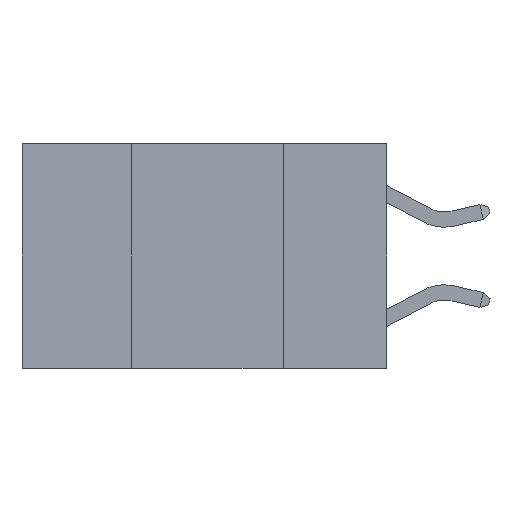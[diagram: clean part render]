
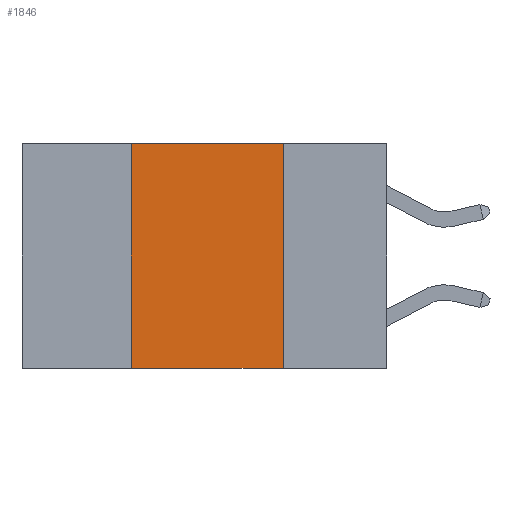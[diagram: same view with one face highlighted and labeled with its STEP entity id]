
A CAD part, left-side view. The second image highlights one B-rep face of the part: STEP entity #1846.
In plain terms, the highlighted planar face has unit normal (-1, 0, 0).
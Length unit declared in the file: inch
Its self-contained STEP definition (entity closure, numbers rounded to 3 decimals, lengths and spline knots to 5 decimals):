
#868 = VERTEX_POINT ( 'NONE', #14202 ) ;
#1846 = ADVANCED_FACE ( 'NONE', ( #6847 ), #14519, .F. ) ;
#1877 = CARTESIAN_POINT ( 'NONE',  ( 0., 0.17, -0.37 ) ) ;
#2147 = DIRECTION ( 'NONE',  ( 0., 0., -1. ) ) ;
#2513 = CARTESIAN_POINT ( 'NONE',  ( 0., 0.42, -0.37 ) ) ;
#3823 = DIRECTION ( 'NONE',  ( 1., 0., 0. ) ) ;
#4658 = VECTOR ( 'NONE', #18278, 39.37008 ) ;
#5845 = CARTESIAN_POINT ( 'NONE',  ( 0., 0.6, -0.37 ) ) ;
#6337 = EDGE_LOOP ( 'NONE', ( #6702, #12960, #11256, #19121 ) ) ;
#6382 = AXIS2_PLACEMENT_3D ( 'NONE', #19244, #3823, #11397 ) ;
#6588 = CARTESIAN_POINT ( 'NONE',  ( 0., 0.6, 0. ) ) ;
#6702 = ORIENTED_EDGE ( 'NONE', *, *, #11040, .F. ) ;
#6831 = EDGE_CURVE ( 'NONE', #8887, #18956, #12034, .T. ) ;
#6847 = FACE_OUTER_BOUND ( 'NONE', #6337, .T. ) ;
#7530 = VECTOR ( 'NONE', #14833, 39.37008 ) ;
#7771 = VERTEX_POINT ( 'NONE', #1877 ) ;
#8114 = LINE ( 'NONE', #18888, #12507 ) ;
#8500 = DIRECTION ( 'NONE',  ( 0., -1., 0. ) ) ;
#8887 = VERTEX_POINT ( 'NONE', #2513 ) ;
#9405 = VECTOR ( 'NONE', #8500, 39.37008 ) ;
#11040 = EDGE_CURVE ( 'NONE', #868, #7771, #8114, .T. ) ;
#11256 = ORIENTED_EDGE ( 'NONE', *, *, #6831, .F. ) ;
#11397 = DIRECTION ( 'NONE',  ( 0., 0., -1. ) ) ;
#12034 = LINE ( 'NONE', #13439, #4658 ) ;
#12507 = VECTOR ( 'NONE', #2147, 39.37008 ) ;
#12960 = ORIENTED_EDGE ( 'NONE', *, *, #16916, .F. ) ;
#13023 = LINE ( 'NONE', #6588, #9405 ) ;
#13439 = CARTESIAN_POINT ( 'NONE',  ( 0., 0.42, 0. ) ) ;
#14202 = CARTESIAN_POINT ( 'NONE',  ( 0., 0.17, 0. ) ) ;
#14519 = PLANE ( 'NONE',  #6382 ) ;
#14833 = DIRECTION ( 'NONE',  ( 0., -1., 0. ) ) ;
#16916 = EDGE_CURVE ( 'NONE', #18956, #868, #13023, .T. ) ;
#17723 = CARTESIAN_POINT ( 'NONE',  ( 0., 0.42, 0. ) ) ;
#18278 = DIRECTION ( 'NONE',  ( 0., 0., 1. ) ) ;
#18769 = EDGE_CURVE ( 'NONE', #8887, #7771, #19669, .T. ) ;
#18888 = CARTESIAN_POINT ( 'NONE',  ( 0., 0.17, 0. ) ) ;
#18956 = VERTEX_POINT ( 'NONE', #17723 ) ;
#19121 = ORIENTED_EDGE ( 'NONE', *, *, #18769, .T. ) ;
#19244 = CARTESIAN_POINT ( 'NONE',  ( 0., 0.6, 0. ) ) ;
#19669 = LINE ( 'NONE', #5845, #7530 ) ;
